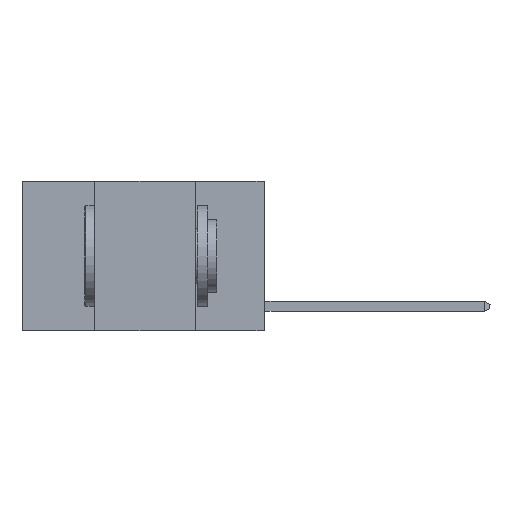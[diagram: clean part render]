
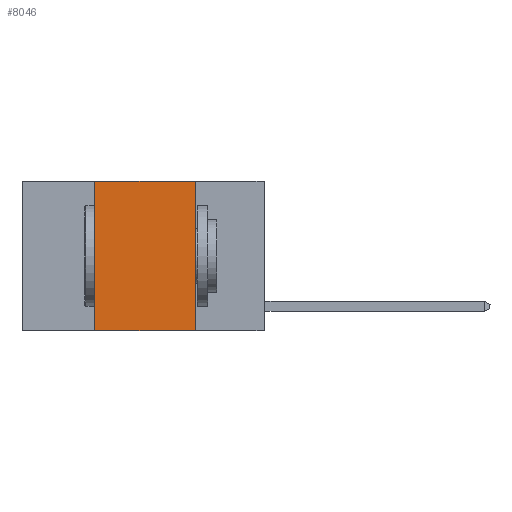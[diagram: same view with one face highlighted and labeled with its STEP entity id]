
A CAD part, left-side view. The second image highlights one B-rep face of the part: STEP entity #8046.
In plain terms, the highlighted planar face has unit normal (-1, 0, 0).
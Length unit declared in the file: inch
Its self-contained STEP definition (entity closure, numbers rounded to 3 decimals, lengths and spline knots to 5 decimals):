
#34 = VERTEX_POINT ( 'NONE', #6095 ) ;
#104 = EDGE_CURVE ( 'NONE', #3360, #14773, #23182, .T. ) ;
#867 = AXIS2_PLACEMENT_3D ( 'NONE', #5840, #18636, #5936 ) ;
#1708 = PLANE ( 'NONE',  #867 ) ;
#2897 = VECTOR ( 'NONE', #6253, 39.37008 ) ;
#3024 = CARTESIAN_POINT ( 'NONE',  ( 0., 0.6, 0. ) ) ;
#3360 = VERTEX_POINT ( 'NONE', #20395 ) ;
#4113 = LINE ( 'NONE', #21795, #9772 ) ;
#4206 = CARTESIAN_POINT ( 'NONE',  ( 0., 0.17, -0.37 ) ) ;
#4323 = VERTEX_POINT ( 'NONE', #6535 ) ;
#4537 = EDGE_CURVE ( 'NONE', #34, #3360, #18070, .T. ) ;
#4833 = DIRECTION ( 'NONE',  ( 0., 0., 1. ) ) ;
#5117 = EDGE_CURVE ( 'NONE', #4323, #34, #4113, .T. ) ;
#5145 = DIRECTION ( 'NONE',  ( 0., -1., 0. ) ) ;
#5840 = CARTESIAN_POINT ( 'NONE',  ( 0., 0.6, 0. ) ) ;
#5936 = DIRECTION ( 'NONE',  ( 0., 0., -1. ) ) ;
#6095 = CARTESIAN_POINT ( 'NONE',  ( 0., 0.42, 0. ) ) ;
#6253 = DIRECTION ( 'NONE',  ( 0., -1., 0. ) ) ;
#6535 = CARTESIAN_POINT ( 'NONE',  ( 0., 0.42, -0.37 ) ) ;
#6798 = VECTOR ( 'NONE', #5145, 39.37008 ) ;
#8046 = ADVANCED_FACE ( 'NONE', ( #8079 ), #1708, .F. ) ;
#8079 = FACE_OUTER_BOUND ( 'NONE', #18103, .T. ) ;
#8491 = DIRECTION ( 'NONE',  ( 0., 0., -1. ) ) ;
#9772 = VECTOR ( 'NONE', #4833, 39.37008 ) ;
#11448 = ORIENTED_EDGE ( 'NONE', *, *, #5117, .F. ) ;
#12583 = VECTOR ( 'NONE', #8491, 39.37008 ) ;
#14773 = VERTEX_POINT ( 'NONE', #4206 ) ;
#15730 = ORIENTED_EDGE ( 'NONE', *, *, #104, .F. ) ;
#16376 = ORIENTED_EDGE ( 'NONE', *, *, #4537, .F. ) ;
#17711 = ORIENTED_EDGE ( 'NONE', *, *, #19023, .T. ) ;
#18070 = LINE ( 'NONE', #3024, #6798 ) ;
#18103 = EDGE_LOOP ( 'NONE', ( #15730, #16376, #11448, #17711 ) ) ;
#18636 = DIRECTION ( 'NONE',  ( 1., 0., 0. ) ) ;
#19023 = EDGE_CURVE ( 'NONE', #4323, #14773, #19797, .T. ) ;
#19797 = LINE ( 'NONE', #21081, #2897 ) ;
#20395 = CARTESIAN_POINT ( 'NONE',  ( 0., 0.17, 0. ) ) ;
#21081 = CARTESIAN_POINT ( 'NONE',  ( 0., 0.6, -0.37 ) ) ;
#21795 = CARTESIAN_POINT ( 'NONE',  ( 0., 0.42, 0. ) ) ;
#23182 = LINE ( 'NONE', #26340, #12583 ) ;
#26340 = CARTESIAN_POINT ( 'NONE',  ( 0., 0.17, 0. ) ) ;
